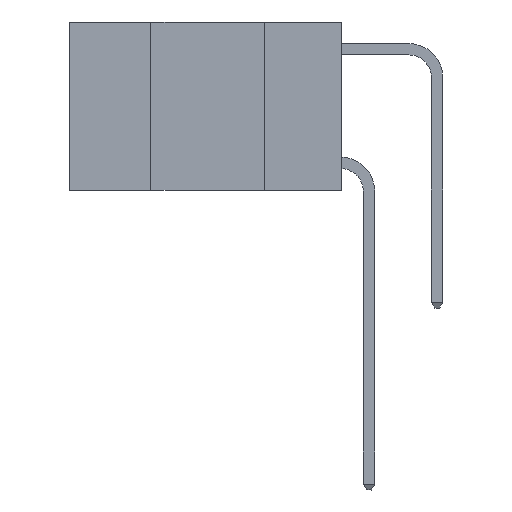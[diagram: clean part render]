
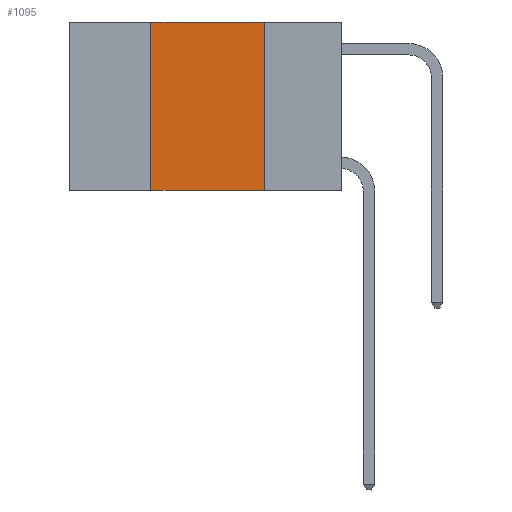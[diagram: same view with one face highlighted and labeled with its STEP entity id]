
A CAD part, left-side view. The second image highlights one B-rep face of the part: STEP entity #1095.
In plain terms, the highlighted planar face has unit normal (-1, 0, 0).
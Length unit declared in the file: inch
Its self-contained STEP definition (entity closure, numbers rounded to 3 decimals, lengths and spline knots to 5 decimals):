
#134 = PLANE ( 'NONE',  #7078 ) ;
#1095 = ADVANCED_FACE ( 'NONE', ( #6344 ), #134, .F. ) ;
#1408 = DIRECTION ( 'NONE',  ( 0., 0., -1. ) ) ;
#1476 = EDGE_CURVE ( 'NONE', #7817, #2331, #7937, .T. ) ;
#1549 = DIRECTION ( 'NONE',  ( 0., 0., -1. ) ) ;
#1706 = EDGE_CURVE ( 'NONE', #2044, #10516, #5861, .T. ) ;
#1961 = CARTESIAN_POINT ( 'NONE',  ( 0., 0.17, 0. ) ) ;
#2044 = VERTEX_POINT ( 'NONE', #8301 ) ;
#2331 = VERTEX_POINT ( 'NONE', #1961 ) ;
#2828 = VECTOR ( 'NONE', #12988, 39.37008 ) ;
#3091 = ORIENTED_EDGE ( 'NONE', *, *, #10535, .F. ) ;
#3466 = VECTOR ( 'NONE', #1549, 39.37008 ) ;
#4473 = ORIENTED_EDGE ( 'NONE', *, *, #1706, .T. ) ;
#4887 = LINE ( 'NONE', #10903, #3466 ) ;
#5402 = DIRECTION ( 'NONE',  ( 0., 0., 1. ) ) ;
#5508 = ORIENTED_EDGE ( 'NONE', *, *, #12329, .F. ) ;
#5861 = LINE ( 'NONE', #10073, #2828 ) ;
#6344 = FACE_OUTER_BOUND ( 'NONE', #10928, .T. ) ;
#6696 = CARTESIAN_POINT ( 'NONE',  ( 0., 0.6, 0. ) ) ;
#6951 = DIRECTION ( 'NONE',  ( 0., -1., 0. ) ) ;
#7078 = AXIS2_PLACEMENT_3D ( 'NONE', #11496, #10574, #1408 ) ;
#7817 = VERTEX_POINT ( 'NONE', #12806 ) ;
#7937 = LINE ( 'NONE', #6696, #9879 ) ;
#8301 = CARTESIAN_POINT ( 'NONE',  ( 0., 0.42, -0.37 ) ) ;
#9008 = VECTOR ( 'NONE', #5402, 39.37008 ) ;
#9879 = VECTOR ( 'NONE', #6951, 39.37008 ) ;
#10073 = CARTESIAN_POINT ( 'NONE',  ( 0., 0.6, -0.37 ) ) ;
#10516 = VERTEX_POINT ( 'NONE', #12448 ) ;
#10535 = EDGE_CURVE ( 'NONE', #2331, #10516, #4887, .T. ) ;
#10574 = DIRECTION ( 'NONE',  ( 1., 0., 0. ) ) ;
#10903 = CARTESIAN_POINT ( 'NONE',  ( 0., 0.17, 0. ) ) ;
#10928 = EDGE_LOOP ( 'NONE', ( #3091, #12528, #5508, #4473 ) ) ;
#11492 = CARTESIAN_POINT ( 'NONE',  ( 0., 0.42, 0. ) ) ;
#11496 = CARTESIAN_POINT ( 'NONE',  ( 0., 0.6, 0. ) ) ;
#11735 = LINE ( 'NONE', #11492, #9008 ) ;
#12329 = EDGE_CURVE ( 'NONE', #2044, #7817, #11735, .T. ) ;
#12448 = CARTESIAN_POINT ( 'NONE',  ( 0., 0.17, -0.37 ) ) ;
#12528 = ORIENTED_EDGE ( 'NONE', *, *, #1476, .F. ) ;
#12806 = CARTESIAN_POINT ( 'NONE',  ( 0., 0.42, 0. ) ) ;
#12988 = DIRECTION ( 'NONE',  ( 0., -1., 0. ) ) ;
